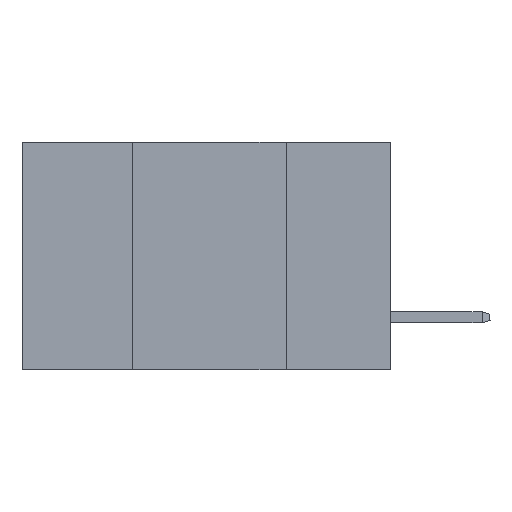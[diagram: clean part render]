
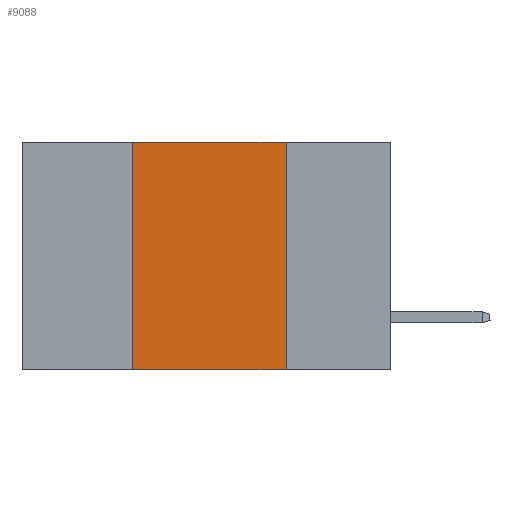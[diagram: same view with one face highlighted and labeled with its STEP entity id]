
A CAD part, left-side view. The second image highlights one B-rep face of the part: STEP entity #9088.
In plain terms, the highlighted planar face has unit normal (-1, 0, 0).
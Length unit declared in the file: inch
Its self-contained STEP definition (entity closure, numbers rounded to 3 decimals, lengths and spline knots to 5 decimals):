
#1071 = VERTEX_POINT ( 'NONE', #13284 ) ;
#2492 = AXIS2_PLACEMENT_3D ( 'NONE', #8620, #18887, #10132 ) ;
#3536 = DIRECTION ( 'NONE',  ( 0., 0., 1. ) ) ;
#4063 = PLANE ( 'NONE',  #2492 ) ;
#4729 = VECTOR ( 'NONE', #6703, 39.37008 ) ;
#5010 = CARTESIAN_POINT ( 'NONE',  ( 0., 0.6, -0.37 ) ) ;
#6122 = CARTESIAN_POINT ( 'NONE',  ( 0., 0.6, 0. ) ) ;
#6266 = EDGE_CURVE ( 'NONE', #1071, #15607, #14250, .T. ) ;
#6669 = CARTESIAN_POINT ( 'NONE',  ( 0., 0.17, -0.37 ) ) ;
#6703 = DIRECTION ( 'NONE',  ( 0., 0., -1. ) ) ;
#6910 = LINE ( 'NONE', #8028, #10418 ) ;
#7169 = VECTOR ( 'NONE', #12125, 39.37008 ) ;
#7777 = CARTESIAN_POINT ( 'NONE',  ( 0., 0.17, 0. ) ) ;
#7929 = EDGE_LOOP ( 'NONE', ( #13435, #8073, #17208, #11521 ) ) ;
#8028 = CARTESIAN_POINT ( 'NONE',  ( 0., 0.42, 0. ) ) ;
#8073 = ORIENTED_EDGE ( 'NONE', *, *, #6266, .F. ) ;
#8620 = CARTESIAN_POINT ( 'NONE',  ( 0., 0.6, 0. ) ) ;
#9088 = ADVANCED_FACE ( 'NONE', ( #11390 ), #4063, .F. ) ;
#10132 = DIRECTION ( 'NONE',  ( 0., 0., -1. ) ) ;
#10383 = VECTOR ( 'NONE', #12080, 39.37008 ) ;
#10418 = VECTOR ( 'NONE', #3536, 39.37008 ) ;
#10836 = EDGE_CURVE ( 'NONE', #17429, #15780, #18903, .T. ) ;
#11390 = FACE_OUTER_BOUND ( 'NONE', #7929, .T. ) ;
#11521 = ORIENTED_EDGE ( 'NONE', *, *, #10836, .T. ) ;
#12029 = CARTESIAN_POINT ( 'NONE',  ( 0., 0.42, -0.37 ) ) ;
#12072 = EDGE_CURVE ( 'NONE', #17429, #1071, #6910, .T. ) ;
#12080 = DIRECTION ( 'NONE',  ( 0., -1., 0. ) ) ;
#12125 = DIRECTION ( 'NONE',  ( 0., -1., 0. ) ) ;
#12798 = EDGE_CURVE ( 'NONE', #15607, #15780, #17021, .T. ) ;
#13284 = CARTESIAN_POINT ( 'NONE',  ( 0., 0.42, 0. ) ) ;
#13435 = ORIENTED_EDGE ( 'NONE', *, *, #12798, .F. ) ;
#14250 = LINE ( 'NONE', #6122, #10383 ) ;
#15607 = VERTEX_POINT ( 'NONE', #7777 ) ;
#15780 = VERTEX_POINT ( 'NONE', #6669 ) ;
#17003 = CARTESIAN_POINT ( 'NONE',  ( 0., 0.17, 0. ) ) ;
#17021 = LINE ( 'NONE', #17003, #4729 ) ;
#17208 = ORIENTED_EDGE ( 'NONE', *, *, #12072, .F. ) ;
#17429 = VERTEX_POINT ( 'NONE', #12029 ) ;
#18887 = DIRECTION ( 'NONE',  ( 1., 0., 0. ) ) ;
#18903 = LINE ( 'NONE', #5010, #7169 ) ;
